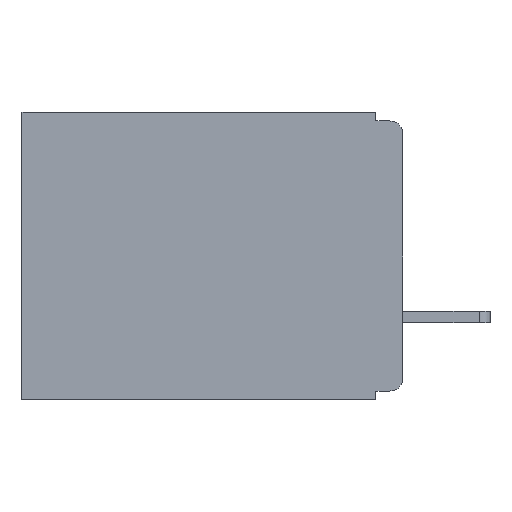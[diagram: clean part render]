
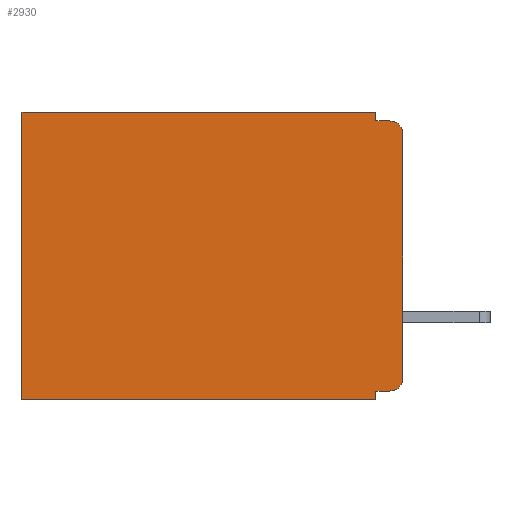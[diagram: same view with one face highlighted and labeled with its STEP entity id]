
A CAD part, left-side view. The second image highlights one B-rep face of the part: STEP entity #2930.
In plain terms, the highlighted planar face has unit normal (-1, 0, 0).
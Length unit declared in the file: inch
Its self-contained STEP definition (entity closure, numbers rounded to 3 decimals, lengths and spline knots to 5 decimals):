
#152 = CIRCLE ( 'NONE', #7900, 0.015 ) ;
#195 = VERTEX_POINT ( 'NONE', #398 ) ;
#392 = ORIENTED_EDGE ( 'NONE', *, *, #6181, .F. ) ;
#398 = CARTESIAN_POINT ( 'NONE',  ( 0.3, 0.015, -0.01 ) ) ;
#437 = AXIS2_PLACEMENT_3D ( 'NONE', #6646, #7314, #12012 ) ;
#607 = CARTESIAN_POINT ( 'NONE',  ( 0.3, 0.437, -0.33 ) ) ;
#669 = DIRECTION ( 'NONE',  ( 1., 0., 0. ) ) ;
#693 = VERTEX_POINT ( 'NONE', #7985 ) ;
#707 = VERTEX_POINT ( 'NONE', #8156 ) ;
#744 = CARTESIAN_POINT ( 'NONE',  ( 0.3, 0., -0.025 ) ) ;
#931 = DIRECTION ( 'NONE',  ( 0., 0., -1. ) ) ;
#1032 = DIRECTION ( 'NONE',  ( 0., 1., 0. ) ) ;
#1095 = CARTESIAN_POINT ( 'NONE',  ( 0.3, 0.031, -0.01 ) ) ;
#1215 = AXIS2_PLACEMENT_3D ( 'NONE', #7006, #669, #9400 ) ;
#1320 = VECTOR ( 'NONE', #9601, 39.37008 ) ;
#1566 = CARTESIAN_POINT ( 'NONE',  ( 0.3, 0.031, -0.32 ) ) ;
#1660 = DIRECTION ( 'NONE',  ( 0., -1., 0. ) ) ;
#1690 = CARTESIAN_POINT ( 'NONE',  ( 0.3, 0., -0.01 ) ) ;
#2930 = ADVANCED_FACE ( 'NONE', ( #12444 ), #7508, .F. ) ;
#3550 = VERTEX_POINT ( 'NONE', #6462 ) ;
#3941 = VERTEX_POINT ( 'NONE', #12750 ) ;
#4138 = VECTOR ( 'NONE', #1032, 39.37008 ) ;
#4296 = CIRCLE ( 'NONE', #437, 0.015 ) ;
#5213 = LINE ( 'NONE', #13198, #11005 ) ;
#5701 = EDGE_CURVE ( 'NONE', #3550, #10686, #10330, .T. ) ;
#5705 = EDGE_CURVE ( 'NONE', #11232, #3941, #13204, .T. ) ;
#5969 = DIRECTION ( 'NONE',  ( 0., 0., -1. ) ) ;
#6046 = EDGE_LOOP ( 'NONE', ( #10770, #7722, #392, #6339, #12079, #9101, #11729, #14390, #11639, #10950 ) ) ;
#6181 = EDGE_CURVE ( 'NONE', #11945, #195, #10820, .T. ) ;
#6339 = ORIENTED_EDGE ( 'NONE', *, *, #11080, .F. ) ;
#6462 = CARTESIAN_POINT ( 'NONE',  ( 0.3, 0.031, 0. ) ) ;
#6476 = EDGE_CURVE ( 'NONE', #707, #12629, #5213, .T. ) ;
#6558 = LINE ( 'NONE', #607, #9338 ) ;
#6625 = EDGE_CURVE ( 'NONE', #11232, #195, #152, .T. ) ;
#6646 = CARTESIAN_POINT ( 'NONE',  ( 0.3, 0.015, -0.305 ) ) ;
#6670 = LINE ( 'NONE', #13138, #14731 ) ;
#6736 = EDGE_CURVE ( 'NONE', #707, #3941, #4296, .T. ) ;
#6834 = CARTESIAN_POINT ( 'NONE',  ( 0.3, 0.015, -0.025 ) ) ;
#7006 = CARTESIAN_POINT ( 'NONE',  ( 0.3, 0., -0.33 ) ) ;
#7314 = DIRECTION ( 'NONE',  ( -1., 0., 0. ) ) ;
#7407 = VECTOR ( 'NONE', #1660, 39.37008 ) ;
#7461 = LINE ( 'NONE', #8061, #13067 ) ;
#7508 = PLANE ( 'NONE',  #1215 ) ;
#7722 = ORIENTED_EDGE ( 'NONE', *, *, #6625, .T. ) ;
#7900 = AXIS2_PLACEMENT_3D ( 'NONE', #6834, #8086, #12911 ) ;
#7985 = CARTESIAN_POINT ( 'NONE',  ( 0.3, 0.437, -0.33 ) ) ;
#8061 = CARTESIAN_POINT ( 'NONE',  ( 0.3, 0., -0.33 ) ) ;
#8086 = DIRECTION ( 'NONE',  ( -1., 0., 0. ) ) ;
#8156 = CARTESIAN_POINT ( 'NONE',  ( 0.3, 0.015, -0.32 ) ) ;
#8423 = CARTESIAN_POINT ( 'NONE',  ( 0.3, 0.031, -0.33 ) ) ;
#8500 = VERTEX_POINT ( 'NONE', #9581 ) ;
#8741 = EDGE_CURVE ( 'NONE', #10686, #693, #6558, .T. ) ;
#8975 = DIRECTION ( 'NONE',  ( 0., 1., 0. ) ) ;
#9101 = ORIENTED_EDGE ( 'NONE', *, *, #8741, .T. ) ;
#9246 = DIRECTION ( 'NONE',  ( 0., 1., 0. ) ) ;
#9338 = VECTOR ( 'NONE', #931, 39.37008 ) ;
#9400 = DIRECTION ( 'NONE',  ( 0., 0., -1. ) ) ;
#9581 = CARTESIAN_POINT ( 'NONE',  ( 0.3, 0.031, -0.33 ) ) ;
#9601 = DIRECTION ( 'NONE',  ( 0., 0., -1. ) ) ;
#9805 = EDGE_CURVE ( 'NONE', #8500, #693, #7461, .T. ) ;
#9948 = EDGE_CURVE ( 'NONE', #12629, #8500, #10697, .T. ) ;
#9982 = VECTOR ( 'NONE', #5969, 39.37008 ) ;
#10330 = LINE ( 'NONE', #12166, #4138 ) ;
#10686 = VERTEX_POINT ( 'NONE', #14293 ) ;
#10697 = LINE ( 'NONE', #8423, #1320 ) ;
#10770 = ORIENTED_EDGE ( 'NONE', *, *, #5705, .F. ) ;
#10820 = LINE ( 'NONE', #1690, #7407 ) ;
#10950 = ORIENTED_EDGE ( 'NONE', *, *, #6736, .T. ) ;
#11005 = VECTOR ( 'NONE', #8975, 39.37008 ) ;
#11080 = EDGE_CURVE ( 'NONE', #3550, #11945, #6670, .T. ) ;
#11232 = VERTEX_POINT ( 'NONE', #744 ) ;
#11639 = ORIENTED_EDGE ( 'NONE', *, *, #6476, .F. ) ;
#11729 = ORIENTED_EDGE ( 'NONE', *, *, #9805, .F. ) ;
#11945 = VERTEX_POINT ( 'NONE', #1095 ) ;
#12012 = DIRECTION ( 'NONE',  ( 0., 0., -1. ) ) ;
#12079 = ORIENTED_EDGE ( 'NONE', *, *, #5701, .T. ) ;
#12166 = CARTESIAN_POINT ( 'NONE',  ( 0.3, 0., 0. ) ) ;
#12429 = CARTESIAN_POINT ( 'NONE',  ( 0.3, 0., -0.33 ) ) ;
#12444 = FACE_OUTER_BOUND ( 'NONE', #6046, .T. ) ;
#12629 = VERTEX_POINT ( 'NONE', #1566 ) ;
#12750 = CARTESIAN_POINT ( 'NONE',  ( 0.3, 0., -0.305 ) ) ;
#12911 = DIRECTION ( 'NONE',  ( 0., 0., -1. ) ) ;
#13067 = VECTOR ( 'NONE', #9246, 39.37008 ) ;
#13138 = CARTESIAN_POINT ( 'NONE',  ( 0.3, 0.031, 0. ) ) ;
#13198 = CARTESIAN_POINT ( 'NONE',  ( 0.3, 0., -0.32 ) ) ;
#13204 = LINE ( 'NONE', #12429, #9982 ) ;
#14164 = DIRECTION ( 'NONE',  ( 0., 0., -1. ) ) ;
#14293 = CARTESIAN_POINT ( 'NONE',  ( 0.3, 0.437, 0. ) ) ;
#14390 = ORIENTED_EDGE ( 'NONE', *, *, #9948, .F. ) ;
#14731 = VECTOR ( 'NONE', #14164, 39.37008 ) ;
